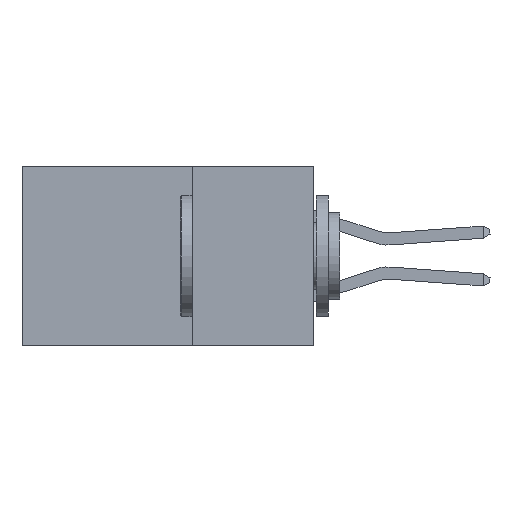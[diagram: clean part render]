
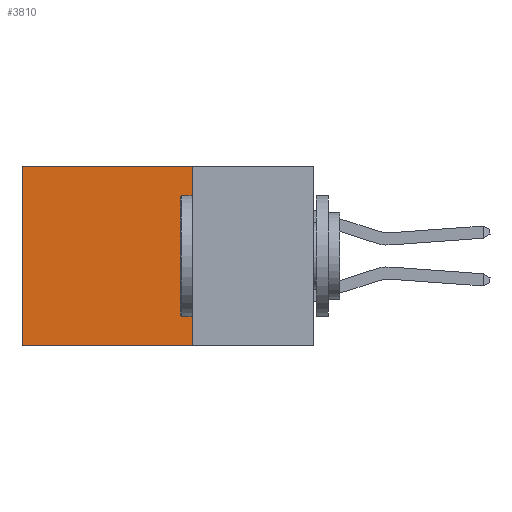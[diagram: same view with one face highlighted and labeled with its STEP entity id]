
A CAD part, left-side view. The second image highlights one B-rep face of the part: STEP entity #3810.
In plain terms, the highlighted planar face has unit normal (-1, 0, 0).
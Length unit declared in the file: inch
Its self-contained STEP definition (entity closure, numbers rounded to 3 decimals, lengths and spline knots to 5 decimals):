
#2263 = LINE ( 'NONE', #24640, #2784 ) ;
#2784 = VECTOR ( 'NONE', #21805, 39.37008 ) ;
#3810 = ADVANCED_FACE ( 'NONE', ( #19898 ), #8422, .F. ) ;
#5848 = VERTEX_POINT ( 'NONE', #17188 ) ;
#7194 = CARTESIAN_POINT ( 'NONE',  ( 0.2875, 0.6, 0. ) ) ;
#8129 = VERTEX_POINT ( 'NONE', #7194 ) ;
#8309 = ORIENTED_EDGE ( 'NONE', *, *, #14424, .F. ) ;
#8422 = PLANE ( 'NONE',  #11275 ) ;
#9401 = DIRECTION ( 'NONE',  ( 1., 0., 0. ) ) ;
#11275 = AXIS2_PLACEMENT_3D ( 'NONE', #35002, #9401, #22261 ) ;
#11998 = EDGE_CURVE ( 'NONE', #19318, #8129, #23047, .T. ) ;
#14045 = CARTESIAN_POINT ( 'NONE',  ( 0.2875, 0.25, 0. ) ) ;
#14371 = VECTOR ( 'NONE', #36611, 39.37008 ) ;
#14424 = EDGE_CURVE ( 'NONE', #19318, #31179, #21372, .T. ) ;
#17188 = CARTESIAN_POINT ( 'NONE',  ( 0.2875, 0.6, -0.37 ) ) ;
#17718 = ORIENTED_EDGE ( 'NONE', *, *, #30353, .T. ) ;
#18684 = DIRECTION ( 'NONE',  ( 0., 0., -1. ) ) ;
#19318 = VERTEX_POINT ( 'NONE', #39092 ) ;
#19336 = VECTOR ( 'NONE', #18684, 39.37008 ) ;
#19530 = EDGE_CURVE ( 'NONE', #31179, #5848, #2263, .T. ) ;
#19898 = FACE_OUTER_BOUND ( 'NONE', #20198, .T. ) ;
#20198 = EDGE_LOOP ( 'NONE', ( #17718, #24680, #8309, #36529 ) ) ;
#20845 = CARTESIAN_POINT ( 'NONE',  ( 0.2875, 0.25, 0. ) ) ;
#21372 = LINE ( 'NONE', #20845, #19336 ) ;
#21805 = DIRECTION ( 'NONE',  ( 0., 1., 0. ) ) ;
#22261 = DIRECTION ( 'NONE',  ( 0., 0., -1. ) ) ;
#23047 = LINE ( 'NONE', #14045, #14371 ) ;
#23953 = VECTOR ( 'NONE', #25407, 39.37008 ) ;
#24640 = CARTESIAN_POINT ( 'NONE',  ( 0.2875, 0.25, -0.37 ) ) ;
#24680 = ORIENTED_EDGE ( 'NONE', *, *, #19530, .F. ) ;
#25407 = DIRECTION ( 'NONE',  ( 0., 0., -1. ) ) ;
#30353 = EDGE_CURVE ( 'NONE', #8129, #5848, #41219, .T. ) ;
#31179 = VERTEX_POINT ( 'NONE', #36417 ) ;
#34776 = CARTESIAN_POINT ( 'NONE',  ( 0.2875, 0.6, 0. ) ) ;
#35002 = CARTESIAN_POINT ( 'NONE',  ( 0.2875, 0.25, 0. ) ) ;
#36417 = CARTESIAN_POINT ( 'NONE',  ( 0.2875, 0.25, -0.37 ) ) ;
#36529 = ORIENTED_EDGE ( 'NONE', *, *, #11998, .T. ) ;
#36611 = DIRECTION ( 'NONE',  ( 0., 1., 0. ) ) ;
#39092 = CARTESIAN_POINT ( 'NONE',  ( 0.2875, 0.25, 0. ) ) ;
#41219 = LINE ( 'NONE', #34776, #23953 ) ;
